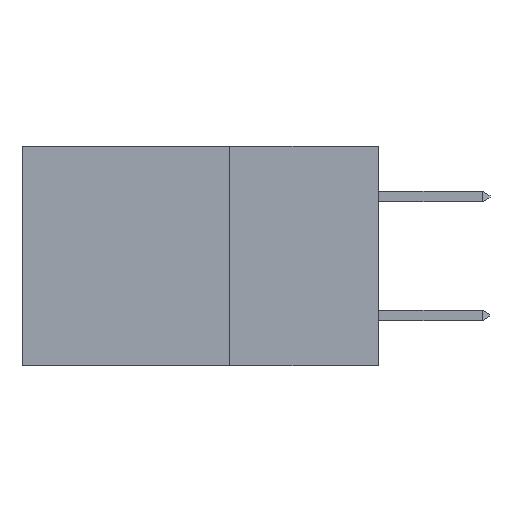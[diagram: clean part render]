
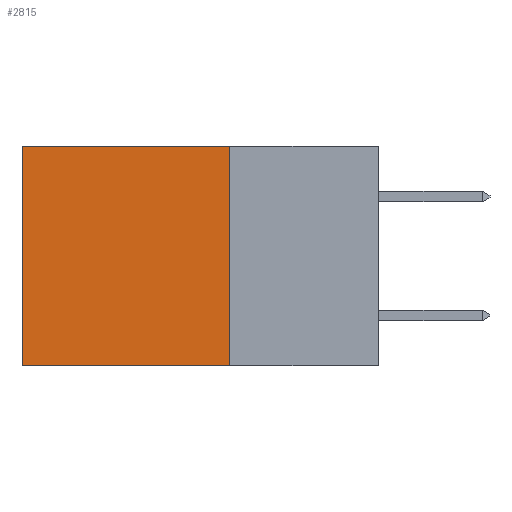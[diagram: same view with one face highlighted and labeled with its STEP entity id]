
A CAD part, left-side view. The second image highlights one B-rep face of the part: STEP entity #2815.
In plain terms, the highlighted planar face has unit normal (-1, 0, 0).
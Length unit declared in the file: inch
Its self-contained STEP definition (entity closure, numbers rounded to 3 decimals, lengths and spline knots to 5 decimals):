
#10 = CARTESIAN_POINT ( 'NONE',  ( 0.298, 0.25, 0. ) ) ;
#150 = CARTESIAN_POINT ( 'NONE',  ( 0.298, 0.25, 0. ) ) ;
#183 = CARTESIAN_POINT ( 'NONE',  ( 0.298, 0.6, 0. ) ) ;
#335 = VECTOR ( 'NONE', #12579, 39.37008 ) ;
#429 = EDGE_LOOP ( 'NONE', ( #11436, #679, #6478, #9205 ) ) ;
#679 = ORIENTED_EDGE ( 'NONE', *, *, #1668, .F. ) ;
#1061 = DIRECTION ( 'NONE',  ( 0., 0., -1. ) ) ;
#1089 = CARTESIAN_POINT ( 'NONE',  ( 0.298, 0.25, 0. ) ) ;
#1668 = EDGE_CURVE ( 'NONE', #9409, #6112, #11735, .T. ) ;
#2494 = EDGE_CURVE ( 'NONE', #10270, #9409, #12791, .T. ) ;
#2815 = ADVANCED_FACE ( 'NONE', ( #3040 ), #10231, .F. ) ;
#2887 = CARTESIAN_POINT ( 'NONE',  ( 0.298, 0.25, -0.37 ) ) ;
#2940 = VERTEX_POINT ( 'NONE', #183 ) ;
#3040 = FACE_OUTER_BOUND ( 'NONE', #429, .T. ) ;
#3313 = DIRECTION ( 'NONE',  ( 0., 1., 0. ) ) ;
#3682 = LINE ( 'NONE', #10, #6199 ) ;
#4351 = CARTESIAN_POINT ( 'NONE',  ( 0.298, 0.6, -0.37 ) ) ;
#5235 = AXIS2_PLACEMENT_3D ( 'NONE', #150, #6235, #7422 ) ;
#6112 = VERTEX_POINT ( 'NONE', #4351 ) ;
#6199 = VECTOR ( 'NONE', #3313, 39.37008 ) ;
#6235 = DIRECTION ( 'NONE',  ( 1., 0., 0. ) ) ;
#6241 = EDGE_CURVE ( 'NONE', #2940, #6112, #6509, .T. ) ;
#6478 = ORIENTED_EDGE ( 'NONE', *, *, #2494, .F. ) ;
#6509 = LINE ( 'NONE', #10562, #11466 ) ;
#7090 = EDGE_CURVE ( 'NONE', #10270, #2940, #3682, .T. ) ;
#7181 = CARTESIAN_POINT ( 'NONE',  ( 0.298, 0.25, 0. ) ) ;
#7422 = DIRECTION ( 'NONE',  ( 0., 0., -1. ) ) ;
#9205 = ORIENTED_EDGE ( 'NONE', *, *, #7090, .T. ) ;
#9409 = VERTEX_POINT ( 'NONE', #2887 ) ;
#10231 = PLANE ( 'NONE',  #5235 ) ;
#10270 = VERTEX_POINT ( 'NONE', #7181 ) ;
#10562 = CARTESIAN_POINT ( 'NONE',  ( 0.298, 0.6, 0. ) ) ;
#11436 = ORIENTED_EDGE ( 'NONE', *, *, #6241, .T. ) ;
#11466 = VECTOR ( 'NONE', #11518, 39.37008 ) ;
#11518 = DIRECTION ( 'NONE',  ( 0., 0., -1. ) ) ;
#11735 = LINE ( 'NONE', #12674, #335 ) ;
#12490 = VECTOR ( 'NONE', #1061, 39.37008 ) ;
#12579 = DIRECTION ( 'NONE',  ( 0., 1., 0. ) ) ;
#12674 = CARTESIAN_POINT ( 'NONE',  ( 0.298, 0.25, -0.37 ) ) ;
#12791 = LINE ( 'NONE', #1089, #12490 ) ;
